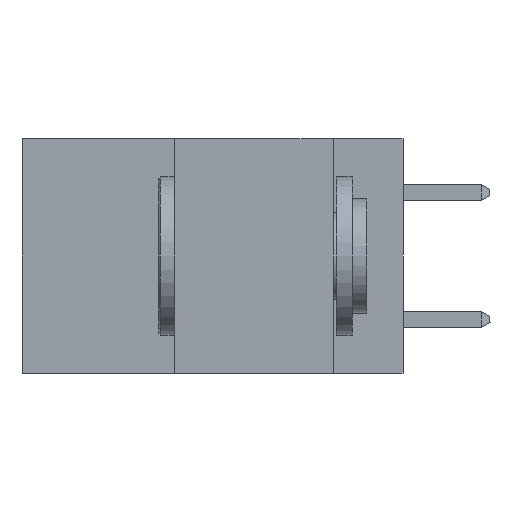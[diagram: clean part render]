
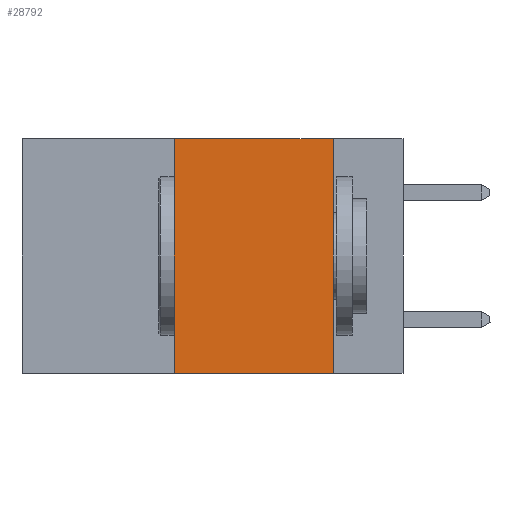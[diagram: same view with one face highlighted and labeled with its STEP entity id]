
A CAD part, left-side view. The second image highlights one B-rep face of the part: STEP entity #28792.
In plain terms, the highlighted planar face has unit normal (-1, 0, 0).
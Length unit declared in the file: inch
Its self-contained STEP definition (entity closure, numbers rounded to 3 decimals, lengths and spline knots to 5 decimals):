
#661 = CARTESIAN_POINT ( 'NONE',  ( 0., 0.36, -0.37 ) ) ;
#1620 = CARTESIAN_POINT ( 'NONE',  ( 0., 0.36, 0. ) ) ;
#2551 = CARTESIAN_POINT ( 'NONE',  ( 0., 0.11, 0. ) ) ;
#2778 = EDGE_LOOP ( 'NONE', ( #8293, #27851, #31297, #33586 ) ) ;
#3298 = VERTEX_POINT ( 'NONE', #1620 ) ;
#3445 = EDGE_CURVE ( 'NONE', #28312, #3298, #18989, .T. ) ;
#3979 = VECTOR ( 'NONE', #18994, 39.37008 ) ;
#4782 = CARTESIAN_POINT ( 'NONE',  ( 0., 0.6, -0.37 ) ) ;
#6551 = AXIS2_PLACEMENT_3D ( 'NONE', #36852, #33345, #11318 ) ;
#6921 = VERTEX_POINT ( 'NONE', #30697 ) ;
#7961 = CARTESIAN_POINT ( 'NONE',  ( 0., 0.6, 0. ) ) ;
#8293 = ORIENTED_EDGE ( 'NONE', *, *, #35172, .F. ) ;
#11318 = DIRECTION ( 'NONE',  ( 0., 0., -1. ) ) ;
#13716 = LINE ( 'NONE', #7961, #3979 ) ;
#18989 = LINE ( 'NONE', #35471, #47046 ) ;
#18994 = DIRECTION ( 'NONE',  ( 0., -1., 0. ) ) ;
#24524 = DIRECTION ( 'NONE',  ( 0., 0., 1. ) ) ;
#27851 = ORIENTED_EDGE ( 'NONE', *, *, #42180, .F. ) ;
#28245 = DIRECTION ( 'NONE',  ( 0., 0., -1. ) ) ;
#28312 = VERTEX_POINT ( 'NONE', #661 ) ;
#28792 = ADVANCED_FACE ( 'NONE', ( #30516 ), #44168, .F. ) ;
#30516 = FACE_OUTER_BOUND ( 'NONE', #2778, .T. ) ;
#30697 = CARTESIAN_POINT ( 'NONE',  ( 0., 0.11, 0. ) ) ;
#31297 = ORIENTED_EDGE ( 'NONE', *, *, #3445, .F. ) ;
#32364 = EDGE_CURVE ( 'NONE', #28312, #37958, #33757, .T. ) ;
#33345 = DIRECTION ( 'NONE',  ( 1., 0., 0. ) ) ;
#33586 = ORIENTED_EDGE ( 'NONE', *, *, #32364, .T. ) ;
#33757 = LINE ( 'NONE', #4782, #43429 ) ;
#34139 = DIRECTION ( 'NONE',  ( 0., -1., 0. ) ) ;
#35172 = EDGE_CURVE ( 'NONE', #6921, #37958, #38110, .T. ) ;
#35471 = CARTESIAN_POINT ( 'NONE',  ( 0., 0.36, 0. ) ) ;
#36852 = CARTESIAN_POINT ( 'NONE',  ( 0., 0.6, 0. ) ) ;
#37958 = VERTEX_POINT ( 'NONE', #41373 ) ;
#38110 = LINE ( 'NONE', #2551, #39264 ) ;
#39264 = VECTOR ( 'NONE', #28245, 39.37008 ) ;
#41373 = CARTESIAN_POINT ( 'NONE',  ( 0., 0.11, -0.37 ) ) ;
#42180 = EDGE_CURVE ( 'NONE', #3298, #6921, #13716, .T. ) ;
#43429 = VECTOR ( 'NONE', #34139, 39.37008 ) ;
#44168 = PLANE ( 'NONE',  #6551 ) ;
#47046 = VECTOR ( 'NONE', #24524, 39.37008 ) ;
